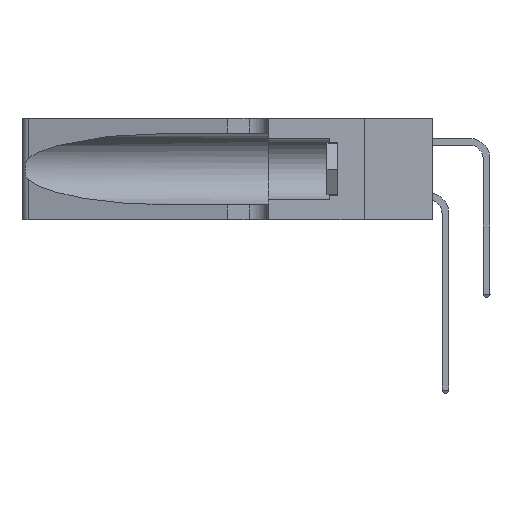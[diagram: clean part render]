
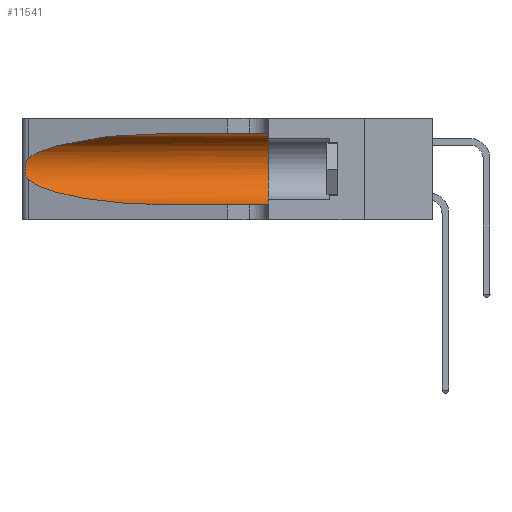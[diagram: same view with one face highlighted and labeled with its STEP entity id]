
A CAD part, left-side view. The second image highlights one B-rep face of the part: STEP entity #11541.
In plain terms, the highlighted cylindrical face has radius 3.308 mm (diameter 6.617 mm), a partial arc.
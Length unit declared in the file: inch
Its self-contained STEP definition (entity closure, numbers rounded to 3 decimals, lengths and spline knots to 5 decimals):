
#251 = CARTESIAN_POINT ( 'NONE',  ( 0.1305, 0.72297, 0.05475 ) ) ;
#677 = CARTESIAN_POINT ( 'NONE',  ( 0.1305, 1.61858, 0.185 ) ) ;
#1320 = CARTESIAN_POINT ( 'NONE',  ( 0.26017, 1.23833, 0.17102 ) ) ;
#1529 = CARTESIAN_POINT ( 'NONE',  ( 0.1305, 1.61858, 0.05475 ) ) ;
#2669 = VERTEX_POINT ( 'NONE', #33341 ) ;
#2767 = CYLINDRICAL_SURFACE ( 'NONE', #13496, 0.13025 ) ;
#3367 = DIRECTION ( 'NONE',  ( 0., -1., 0. ) ) ;
#3787 = CARTESIAN_POINT ( 'NONE',  ( 0.18966, 0.96281, 0.31525 ) ) ;
#4013 = CARTESIAN_POINT ( 'NONE',  ( 0.25789, 1.23486, 0.15765 ) ) ;
#4219 = CARTESIAN_POINT ( 'NONE',  ( 0.1305, 0.35, 0.05475 ) ) ;
#4331 = CARTESIAN_POINT ( 'NONE',  ( 0.2373, 1.15595, 0.08982 ) ) ;
#5844 = VERTEX_POINT ( 'NONE', #251 ) ;
#6194 = EDGE_CURVE ( 'NONE', #7382, #5844, #33757, .T. ) ;
#6312 = CARTESIAN_POINT ( 'NONE',  ( 0.25555, 1.22994, 0.2215 ) ) ;
#6462 = CARTESIAN_POINT ( 'NONE',  ( 0.1305, 0.35, 0.185 ) ) ;
#6655 = CARTESIAN_POINT ( 'NONE',  ( 0.25555, 1.22993, 0.14849 ) ) ;
#7382 = VERTEX_POINT ( 'NONE', #8778 ) ;
#8154 = EDGE_CURVE ( 'NONE', #5844, #23967, #9419, .T. ) ;
#8621 = ORIENTED_EDGE ( 'NONE', *, *, #8154, .T. ) ;
#8778 = CARTESIAN_POINT ( 'NONE',  ( 0.25487, 1.22718, 0.14631 ) ) ;
#9158 = DIRECTION ( 'NONE',  ( 0., 0., 1. ) ) ;
#9277 = VERTEX_POINT ( 'NONE', #13938 ) ;
#9419 = LINE ( 'NONE', #1529, #28851 ) ;
#9436 = EDGE_CURVE ( 'NONE', #23396, #7382, #15521, .T. ) ;
#9683 = CARTESIAN_POINT ( 'NONE',  ( 0.18966, 0.96281, 0.05475 ) ) ;
#10423 = CARTESIAN_POINT ( 'NONE',  ( 0.25487, 1.22718, 0.22369 ) ) ;
#11541 = ADVANCED_FACE ( 'NONE', ( #24000 ), #2767, .F. ) ;
#11823 = EDGE_CURVE ( 'NONE', #9277, #2669, #29646, .T. ) ;
#11957 = CARTESIAN_POINT ( 'NONE',  ( 0.25787, 1.23484, 0.2124 ) ) ;
#13496 = AXIS2_PLACEMENT_3D ( 'NONE', #677, #3367, #16692 ) ;
#13938 = CARTESIAN_POINT ( 'NONE',  ( 0.1305, 0.72297, 0.31525 ) ) ;
#14536 = CARTESIAN_POINT ( 'NONE',  ( 0.2373, 1.15595, 0.28018 ) ) ;
#14645 = CARTESIAN_POINT ( 'NONE',  ( 0.26018, 1.23835, 0.19895 ) ) ;
#14896 = EDGE_CURVE ( 'NONE', #2669, #23967, #26253, .T. ) ;
#15521 = B_SPLINE_CURVE_WITH_KNOTS ( 'NONE', 3,
 ( #22538, #6312, #27756, #11957, #30349, #14645, #32966, #17331, #1320, #20009, #4013, #22645, #6655, #25286 ),
 .UNSPECIFIED., .F., .F.,
 ( 4, 2, 2, 2, 2, 2, 4 ),
 ( 0., 0.00027, 0.00053, 0.00107, 0.0016, 0.00187, 0.00214 ),
 .UNSPECIFIED. ) ;
#15637 = DIRECTION ( 'NONE',  ( 0., -1., 0. ) ) ;
#16692 = DIRECTION ( 'NONE',  ( 0., 0., -1. ) ) ;
#17331 = CARTESIAN_POINT ( 'NONE',  ( 0.26075, 1.23896, 0.178 ) ) ;
#17888 = ORIENTED_EDGE ( 'NONE', *, *, #6194, .T. ) ;
#19705 = ORIENTED_EDGE ( 'NONE', *, *, #11823, .F. ) ;
#19862 = EDGE_LOOP ( 'NONE', ( #33970, #23637, #17888, #8621, #30756, #19705 ) ) ;
#20009 = CARTESIAN_POINT ( 'NONE',  ( 0.25856, 1.23593, 0.16098 ) ) ;
#22538 = CARTESIAN_POINT ( 'NONE',  ( 0.25487, 1.22718, 0.22369 ) ) ;
#22645 = CARTESIAN_POINT ( 'NONE',  ( 0.25639, 1.23186, 0.15144 ) ) ;
#22757 = VECTOR ( 'NONE', #15637, 39.37008 ) ;
#22964 = CARTESIAN_POINT ( 'NONE',  ( 0.25487, 1.22718, 0.14631 ) ) ;
#23327 = EDGE_CURVE ( 'NONE', #9277, #23396, #25250, .T. ) ;
#23396 = VERTEX_POINT ( 'NONE', #10423 ) ;
#23637 = ORIENTED_EDGE ( 'NONE', *, *, #9436, .T. ) ;
#23967 = VERTEX_POINT ( 'NONE', #4219 ) ;
#24000 = FACE_OUTER_BOUND ( 'NONE', #19862, .T. ) ;
#25065 = CARTESIAN_POINT ( 'NONE',  ( 0.1305, 0.72297, 0.31525 ) ) ;
#25087 = DIRECTION ( 'NONE',  ( 0., 1., 0. ) ) ;
#25250 =( BOUNDED_CURVE ( )  B_SPLINE_CURVE ( 3, ( #25065, #3787, #14536, #32866 ),
 .UNSPECIFIED., .F., .F. ) 
 B_SPLINE_CURVE_WITH_KNOTS ( ( 4, 4 ),
 ( 1.5708, 2.84003 ),
 .UNSPECIFIED. ) 
 CURVE ( )  GEOMETRIC_REPRESENTATION_ITEM ( )  RATIONAL_B_SPLINE_CURVE ( ( 1., 0.87, 0.87, 1. ) ) 
 REPRESENTATION_ITEM ( '' )  );
#25286 = CARTESIAN_POINT ( 'NONE',  ( 0.25487, 1.22718, 0.14631 ) ) ;
#26253 = CIRCLE ( 'NONE', #30508, 0.13025 ) ;
#27756 = CARTESIAN_POINT ( 'NONE',  ( 0.25639, 1.23184, 0.21858 ) ) ;
#28178 = CARTESIAN_POINT ( 'NONE',  ( 0.1305, 0.72297, 0.05475 ) ) ;
#28705 = CARTESIAN_POINT ( 'NONE',  ( 0.1305, 1.61858, 0.31525 ) ) ;
#28851 = VECTOR ( 'NONE', #30666, 39.37008 ) ;
#29646 = LINE ( 'NONE', #28705, #22757 ) ;
#30349 = CARTESIAN_POINT ( 'NONE',  ( 0.25854, 1.2359, 0.20912 ) ) ;
#30508 = AXIS2_PLACEMENT_3D ( 'NONE', #6462, #25087, #9158 ) ;
#30666 = DIRECTION ( 'NONE',  ( 0., -1., 0. ) ) ;
#30756 = ORIENTED_EDGE ( 'NONE', *, *, #14896, .F. ) ;
#32866 = CARTESIAN_POINT ( 'NONE',  ( 0.25487, 1.22718, 0.22369 ) ) ;
#32966 = CARTESIAN_POINT ( 'NONE',  ( 0.26075, 1.23896, 0.19203 ) ) ;
#33341 = CARTESIAN_POINT ( 'NONE',  ( 0.1305, 0.35, 0.31525 ) ) ;
#33757 =( BOUNDED_CURVE ( )  B_SPLINE_CURVE ( 3, ( #22964, #4331, #9683, #28178 ),
 .UNSPECIFIED., .F., .F. ) 
 B_SPLINE_CURVE_WITH_KNOTS ( ( 4, 4 ),
 ( 3.44316, 4.71239 ),
 .UNSPECIFIED. ) 
 CURVE ( )  GEOMETRIC_REPRESENTATION_ITEM ( )  RATIONAL_B_SPLINE_CURVE ( ( 1., 0.87, 0.87, 1. ) ) 
 REPRESENTATION_ITEM ( '' )  );
#33970 = ORIENTED_EDGE ( 'NONE', *, *, #23327, .T. ) ;
